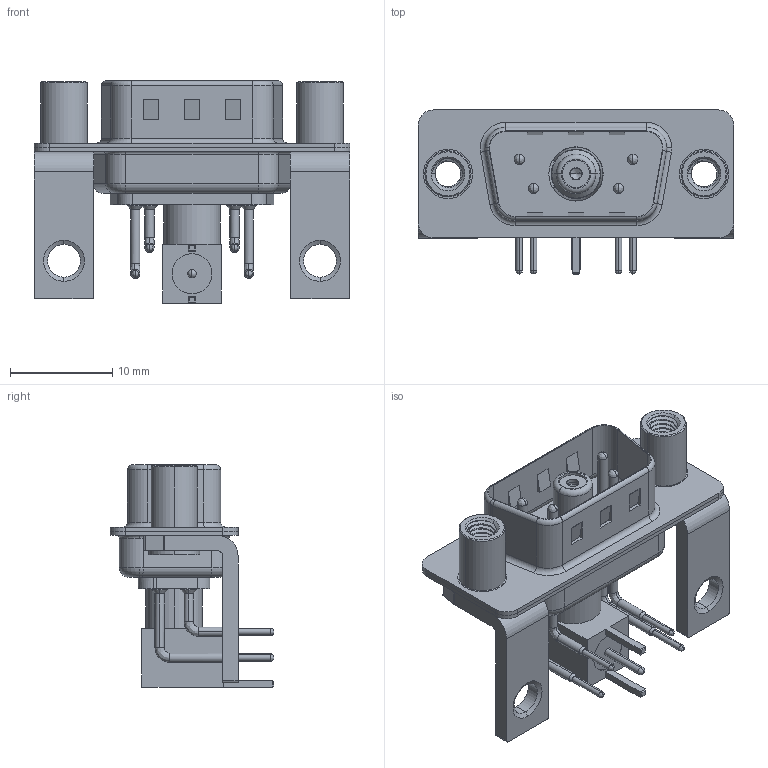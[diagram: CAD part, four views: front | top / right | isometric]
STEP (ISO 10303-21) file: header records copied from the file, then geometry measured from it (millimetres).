
FILE_DESCRIPTION (( 'STEP AP203' ), '1' );
FILE_NAME ('629-5W1-240-7N6.STEP', '2022-05-05T01:05:36', ( '' ), ( '' ), 'SwSTEP 2.0', 'SolidWorks 2020', '' );
FILE_SCHEMA (( 'CONFIG_CONTROL_DESIGN' ));
Length unit declared in the file: millimetre
Products named in the file (16): RA Back Shell; Socket_RA; 629Combo Stabilizer Bracket; Insulator RA Pin; 629Combo Shell Rear_09 Contacts; 629-5W1-240-7N6; Insulator Socket 2; 629Combo Contact Row 1; 629Combo Shell Front_09 Contacts; Co-Ax Jack Assy_RA; Insulator Socket; Locking Collar; 629Combo Housing_5W1; 629Combo Contact Row 2; Co-Ax Jack_RA PC Tail; 629Combo Threaded Standoff_D
Assembly tree (19 placements, depth 3):
  629-5W1-240-7N6
    629Combo Housing_5W1
    629Combo Shell Rear_09 Contacts
    629Combo Shell Front_09 Contacts
    629Combo Stabilizer Bracket  x2
    629Combo Threaded Standoff_D  x2
    Co-Ax Jack Assy_RA
      Co-Ax Jack_RA PC Tail
      Insulator Socket
      Insulator Socket 2
      Locking Collar
      Socket_RA
      RA Back Shell
      Insulator RA Pin
    629Combo Contact Row 1  x2
    629Combo Contact Row 2  x2
Bounding box: 30.8 x 16 x 21.71 mm (x, y, z)
Volume: 2009.6 mm3; surface area: 5540.7 mm2
Topology: 18 solids, 18 shells, 994 faces, 2616 edges, 1677 vertices
Faces by surface type: plane 442, cylinder 412, torus 56, cone 51, bspline 31, sphere 2
Entity records: 25699 total; most frequent: CARTESIAN_POINT 6444, DIRECTION 3778, ORIENTED_EDGE 3588, EDGE_CURVE 1794, AXIS2_PLACEMENT_3D 1377, VERTEX_POINT 1152, VECTOR 1024, LINE 1024
